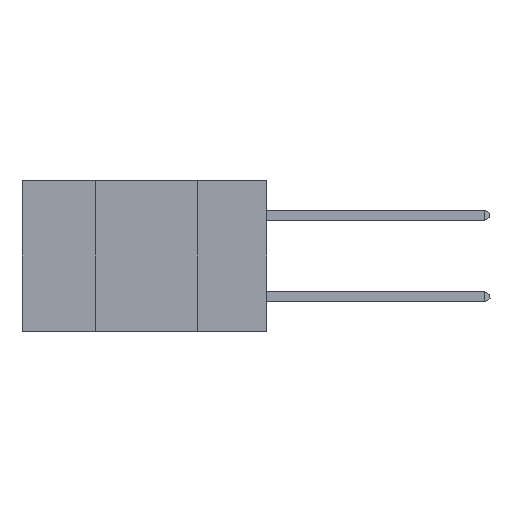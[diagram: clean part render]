
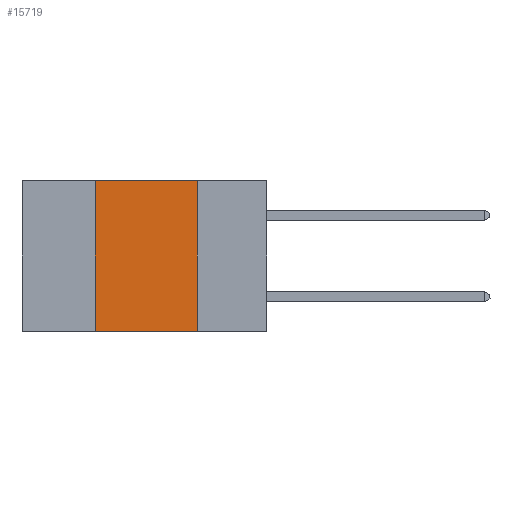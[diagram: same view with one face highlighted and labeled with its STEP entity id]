
A CAD part, left-side view. The second image highlights one B-rep face of the part: STEP entity #15719.
In plain terms, the highlighted planar face has unit normal (-1, 0, 0).
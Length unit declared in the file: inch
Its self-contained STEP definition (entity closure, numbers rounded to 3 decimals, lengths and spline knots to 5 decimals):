
#967 = DIRECTION ( 'NONE',  ( 1., 0., 0. ) ) ;
#1911 = LINE ( 'NONE', #18431, #19497 ) ;
#2367 = ORIENTED_EDGE ( 'NONE', *, *, #8077, .F. ) ;
#3187 = VERTEX_POINT ( 'NONE', #21308 ) ;
#4639 = CARTESIAN_POINT ( 'NONE',  ( 0., 0.17, -0.37 ) ) ;
#4916 = LINE ( 'NONE', #17093, #12961 ) ;
#5263 = FACE_OUTER_BOUND ( 'NONE', #18451, .T. ) ;
#5313 = VERTEX_POINT ( 'NONE', #17955 ) ;
#6349 = ORIENTED_EDGE ( 'NONE', *, *, #6930, .F. ) ;
#6930 = EDGE_CURVE ( 'NONE', #5313, #3187, #19867, .T. ) ;
#8046 = VERTEX_POINT ( 'NONE', #21903 ) ;
#8077 = EDGE_CURVE ( 'NONE', #8046, #19088, #4916, .T. ) ;
#9041 = DIRECTION ( 'NONE',  ( 0., -1., 0. ) ) ;
#9249 = EDGE_CURVE ( 'NONE', #5313, #19088, #1911, .T. ) ;
#9518 = CARTESIAN_POINT ( 'NONE',  ( 0., 0.6, 0. ) ) ;
#10108 = EDGE_CURVE ( 'NONE', #3187, #8046, #11494, .T. ) ;
#10249 = ORIENTED_EDGE ( 'NONE', *, *, #9249, .T. ) ;
#10366 = DIRECTION ( 'NONE',  ( 0., 0., 1. ) ) ;
#10864 = VECTOR ( 'NONE', #10366, 39.37008 ) ;
#11494 = LINE ( 'NONE', #17540, #14999 ) ;
#12942 = DIRECTION ( 'NONE',  ( 0., 0., -1. ) ) ;
#12961 = VECTOR ( 'NONE', #13673, 39.37008 ) ;
#13673 = DIRECTION ( 'NONE',  ( 0., 0., -1. ) ) ;
#14936 = AXIS2_PLACEMENT_3D ( 'NONE', #9518, #967, #12942 ) ;
#14999 = VECTOR ( 'NONE', #9041, 39.37008 ) ;
#15719 = ADVANCED_FACE ( 'NONE', ( #5263 ), #21285, .F. ) ;
#17093 = CARTESIAN_POINT ( 'NONE',  ( 0., 0.17, 0. ) ) ;
#17132 = CARTESIAN_POINT ( 'NONE',  ( 0., 0.42, 0. ) ) ;
#17540 = CARTESIAN_POINT ( 'NONE',  ( 0., 0.6, 0. ) ) ;
#17955 = CARTESIAN_POINT ( 'NONE',  ( 0., 0.42, -0.37 ) ) ;
#18431 = CARTESIAN_POINT ( 'NONE',  ( 0., 0.6, -0.37 ) ) ;
#18451 = EDGE_LOOP ( 'NONE', ( #2367, #20970, #6349, #10249 ) ) ;
#19088 = VERTEX_POINT ( 'NONE', #4639 ) ;
#19497 = VECTOR ( 'NONE', #20102, 39.37008 ) ;
#19867 = LINE ( 'NONE', #17132, #10864 ) ;
#20102 = DIRECTION ( 'NONE',  ( 0., -1., 0. ) ) ;
#20970 = ORIENTED_EDGE ( 'NONE', *, *, #10108, .F. ) ;
#21285 = PLANE ( 'NONE',  #14936 ) ;
#21308 = CARTESIAN_POINT ( 'NONE',  ( 0., 0.42, 0. ) ) ;
#21903 = CARTESIAN_POINT ( 'NONE',  ( 0., 0.17, 0. ) ) ;
